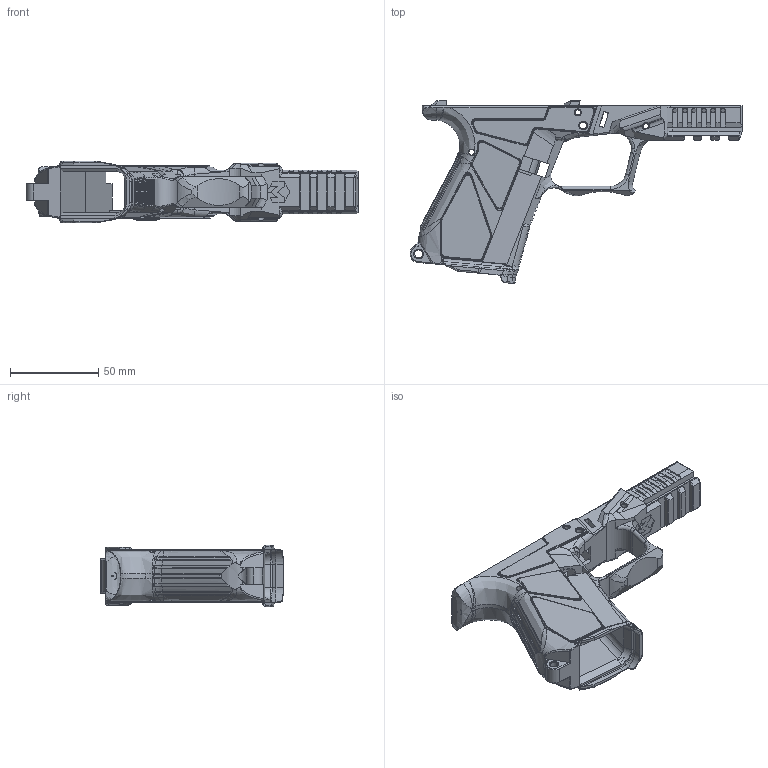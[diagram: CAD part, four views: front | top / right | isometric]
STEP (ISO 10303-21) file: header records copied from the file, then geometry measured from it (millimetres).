
FILE_DESCRIPTION (( 'STEP AP214' ), '1' );
FILE_NAME ('Shnitzle Frame STEP.STEP', '2022-10-03T01:11:03', ( '' ), ( '' ), 'SwSTEP 2.0', 'SolidWorks 2020', '' );
FILE_SCHEMA (( 'AUTOMOTIVE_DESIGN' ));
Length unit declared in the file: inch
Products named in the file (1): Shnitzle Frame STEP
Bounding box: 187.65 x 103.39 x 34.9 mm (x, y, z)
Volume: 93002.1 mm3; surface area: 48871.6 mm2
Topology: 1 solids, 4 shells, 1675 faces, 4471 edges, 2811 vertices
Faces by surface type: plane 687, cylinder 445, bspline 382, cone 72, torus 69, sphere 20
Entity records: 79212 total; most frequent: CARTESIAN_POINT 40958, ORIENTED_EDGE 8936, DIRECTION 6536, EDGE_CURVE 4468, VERTEX_POINT 2811, LINE 2294, VECTOR 2294, AXIS2_PLACEMENT_3D 2121
